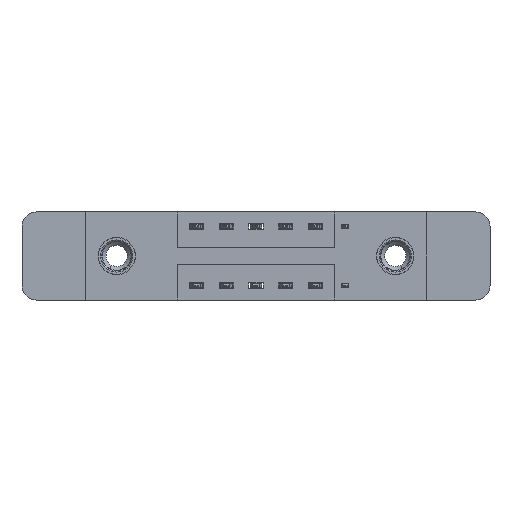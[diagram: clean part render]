
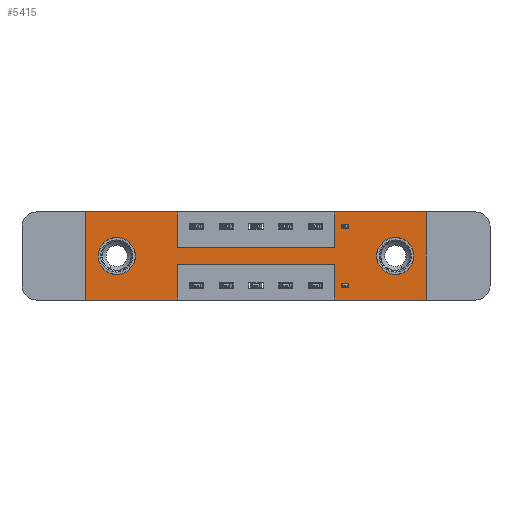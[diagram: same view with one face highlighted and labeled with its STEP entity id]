
A CAD part, front view. The second image highlights one B-rep face of the part: STEP entity #5415.
In plain terms, the highlighted planar face has unit normal (0, -1, 0).
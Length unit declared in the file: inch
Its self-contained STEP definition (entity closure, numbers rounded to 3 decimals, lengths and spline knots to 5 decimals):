
#139 = LINE ( 'NONE', #3190, #13564 ) ;
#177 = CARTESIAN_POINT ( 'NONE',  ( 1.3025, 0., -0.107 ) ) ;
#240 = CARTESIAN_POINT ( 'NONE',  ( 0., 0., -0.37 ) ) ;
#278 = AXIS2_PLACEMENT_3D ( 'NONE', #502, #3787, #12575 ) ;
#338 = VECTOR ( 'NONE', #5071, 39.37008 ) ;
#409 = EDGE_CURVE ( 'NONE', #1438, #1711, #13217, .T. ) ;
#502 = CARTESIAN_POINT ( 'NONE',  ( 1.3025, 0., -0.185 ) ) ;
#896 = EDGE_CURVE ( 'NONE', #1711, #8041, #3485, .T. ) ;
#935 = EDGE_CURVE ( 'NONE', #6880, #13910, #6091, .T. ) ;
#1114 = DIRECTION ( 'NONE',  ( 0., 1., 0. ) ) ;
#1116 = LINE ( 'NONE', #10732, #1658 ) ;
#1154 = DIRECTION ( 'NONE',  ( 0., 0., -1. ) ) ;
#1238 = EDGE_CURVE ( 'NONE', #9080, #6046, #1116, .T. ) ;
#1250 = CARTESIAN_POINT ( 'NONE',  ( 0.3875, 0., -0.15 ) ) ;
#1273 = DIRECTION ( 'NONE',  ( 0., 0., -1. ) ) ;
#1438 = VERTEX_POINT ( 'NONE', #11184 ) ;
#1658 = VECTOR ( 'NONE', #5324, 39.37008 ) ;
#1711 = VERTEX_POINT ( 'NONE', #3855 ) ;
#1749 = VECTOR ( 'NONE', #9826, 39.37008 ) ;
#1819 = ORIENTED_EDGE ( 'NONE', *, *, #8376, .T. ) ;
#1899 = DIRECTION ( 'NONE',  ( 0., 1., 0. ) ) ;
#1933 = CARTESIAN_POINT ( 'NONE',  ( 0., 0., 0. ) ) ;
#2017 = EDGE_CURVE ( 'NONE', #7838, #10262, #11457, .T. ) ;
#2241 = CARTESIAN_POINT ( 'NONE',  ( 1.0475, 0., 0. ) ) ;
#2287 = CARTESIAN_POINT ( 'NONE',  ( 1.0475, 0., -0.15 ) ) ;
#2337 = ORIENTED_EDGE ( 'NONE', *, *, #7295, .T. ) ;
#2591 = DIRECTION ( 'NONE',  ( 1., 0., 0. ) ) ;
#2767 = CARTESIAN_POINT ( 'NONE',  ( 1.435, 0., -0.37 ) ) ;
#2773 = EDGE_CURVE ( 'NONE', #8041, #6880, #8768, .T. ) ;
#2799 = EDGE_CURVE ( 'NONE', #12626, #1438, #139, .T. ) ;
#2966 = CARTESIAN_POINT ( 'NONE',  ( 1.3025, 0., -0.263 ) ) ;
#3064 = VERTEX_POINT ( 'NONE', #177 ) ;
#3154 = CARTESIAN_POINT ( 'NONE',  ( 0., 0., -0.37 ) ) ;
#3190 = CARTESIAN_POINT ( 'NONE',  ( 1.0475, 0., -0.37 ) ) ;
#3387 = LINE ( 'NONE', #240, #10781 ) ;
#3448 = VECTOR ( 'NONE', #5158, 39.37008 ) ;
#3485 = LINE ( 'NONE', #5408, #6715 ) ;
#3629 = DIRECTION ( 'NONE',  ( 0., 0., -1. ) ) ;
#3664 = VECTOR ( 'NONE', #6370, 39.37008 ) ;
#3766 = VERTEX_POINT ( 'NONE', #12826 ) ;
#3787 = DIRECTION ( 'NONE',  ( 0., 1., 0. ) ) ;
#3855 = CARTESIAN_POINT ( 'NONE',  ( 0.3875, 0., -0.22 ) ) ;
#3874 = CARTESIAN_POINT ( 'NONE',  ( 1.0475, 0., -0.37 ) ) ;
#3991 = VECTOR ( 'NONE', #11404, 39.37008 ) ;
#3993 = EDGE_CURVE ( 'NONE', #3766, #13874, #11278, .T. ) ;
#4260 = CARTESIAN_POINT ( 'NONE',  ( 0.1325, 0., -0.263 ) ) ;
#4363 = AXIS2_PLACEMENT_3D ( 'NONE', #8697, #1899, #12703 ) ;
#4497 = ORIENTED_EDGE ( 'NONE', *, *, #3993, .F. ) ;
#4551 = CARTESIAN_POINT ( 'NONE',  ( 1.3025, 0., -0.185 ) ) ;
#5003 = VECTOR ( 'NONE', #2591, 39.37008 ) ;
#5026 = AXIS2_PLACEMENT_3D ( 'NONE', #3154, #7511, #1154 ) ;
#5071 = DIRECTION ( 'NONE',  ( -1., 0., 0. ) ) ;
#5142 = EDGE_LOOP ( 'NONE', ( #1819, #2337 ) ) ;
#5158 = DIRECTION ( 'NONE',  ( 0., 0., -1. ) ) ;
#5266 = CIRCLE ( 'NONE', #4363, 0.078 ) ;
#5279 = FACE_BOUND ( 'NONE', #5142, .T. ) ;
#5324 = DIRECTION ( 'NONE',  ( 1., 0., 0. ) ) ;
#5398 = DIRECTION ( 'NONE',  ( 0., 0., 1. ) ) ;
#5408 = CARTESIAN_POINT ( 'NONE',  ( 0.3875, 0., -0.37 ) ) ;
#5415 = ADVANCED_FACE ( 'NONE', ( #5279, #11534, #9643 ), #12884, .T. ) ;
#5534 = ORIENTED_EDGE ( 'NONE', *, *, #2017, .T. ) ;
#5658 = CARTESIAN_POINT ( 'NONE',  ( 0.1325, 0., -0.107 ) ) ;
#6001 = VERTEX_POINT ( 'NONE', #2767 ) ;
#6046 = VERTEX_POINT ( 'NONE', #11636 ) ;
#6091 = LINE ( 'NONE', #6300, #8064 ) ;
#6149 = LINE ( 'NONE', #11495, #3448 ) ;
#6277 = DIRECTION ( 'NONE',  ( 1., 0., 0. ) ) ;
#6282 = CARTESIAN_POINT ( 'NONE',  ( 0.3875, 0., -0.22 ) ) ;
#6300 = CARTESIAN_POINT ( 'NONE',  ( 0., 0., 0. ) ) ;
#6370 = DIRECTION ( 'NONE',  ( 0., 0., 1. ) ) ;
#6399 = CIRCLE ( 'NONE', #278, 0.078 ) ;
#6680 = DIRECTION ( 'NONE',  ( 0., 0., 1. ) ) ;
#6715 = VECTOR ( 'NONE', #1273, 39.37008 ) ;
#6880 = VERTEX_POINT ( 'NONE', #13185 ) ;
#7243 = DIRECTION ( 'NONE',  ( 0., 0., 1. ) ) ;
#7295 = EDGE_CURVE ( 'NONE', #11156, #3064, #9133, .T. ) ;
#7344 = ORIENTED_EDGE ( 'NONE', *, *, #8258, .F. ) ;
#7386 = AXIS2_PLACEMENT_3D ( 'NONE', #9753, #1114, #6680 ) ;
#7466 = EDGE_CURVE ( 'NONE', #11814, #9080, #11769, .T. ) ;
#7511 = DIRECTION ( 'NONE',  ( 0., -1., 0. ) ) ;
#7545 = AXIS2_PLACEMENT_3D ( 'NONE', #4551, #12349, #3629 ) ;
#7838 = VERTEX_POINT ( 'NONE', #5658 ) ;
#8041 = VERTEX_POINT ( 'NONE', #8097 ) ;
#8064 = VECTOR ( 'NONE', #7243, 39.37008 ) ;
#8097 = CARTESIAN_POINT ( 'NONE',  ( 0.3875, 0., -0.37 ) ) ;
#8100 = LINE ( 'NONE', #1250, #5003 ) ;
#8208 = ORIENTED_EDGE ( 'NONE', *, *, #409, .F. ) ;
#8258 = EDGE_CURVE ( 'NONE', #13910, #3766, #9640, .T. ) ;
#8376 = EDGE_CURVE ( 'NONE', #3064, #11156, #6399, .T. ) ;
#8697 = CARTESIAN_POINT ( 'NONE',  ( 0.1325, 0., -0.185 ) ) ;
#8768 = LINE ( 'NONE', #12122, #1749 ) ;
#8789 = ORIENTED_EDGE ( 'NONE', *, *, #896, .F. ) ;
#8815 = ORIENTED_EDGE ( 'NONE', *, *, #2799, .F. ) ;
#8833 = EDGE_CURVE ( 'NONE', #6046, #6001, #6149, .T. ) ;
#9024 = CARTESIAN_POINT ( 'NONE',  ( 0.3875, 0., 0. ) ) ;
#9080 = VERTEX_POINT ( 'NONE', #11894 ) ;
#9133 = CIRCLE ( 'NONE', #7545, 0.078 ) ;
#9161 = ORIENTED_EDGE ( 'NONE', *, *, #2773, .F. ) ;
#9181 = EDGE_CURVE ( 'NONE', #13874, #11814, #8100, .T. ) ;
#9329 = ORIENTED_EDGE ( 'NONE', *, *, #10178, .T. ) ;
#9640 = LINE ( 'NONE', #1933, #12511 ) ;
#9643 = FACE_OUTER_BOUND ( 'NONE', #11078, .T. ) ;
#9753 = CARTESIAN_POINT ( 'NONE',  ( 0.1325, 0., -0.185 ) ) ;
#9826 = DIRECTION ( 'NONE',  ( -1., 0., 0. ) ) ;
#9962 = ORIENTED_EDGE ( 'NONE', *, *, #935, .F. ) ;
#10178 = EDGE_CURVE ( 'NONE', #10262, #7838, #5266, .T. ) ;
#10262 = VERTEX_POINT ( 'NONE', #4260 ) ;
#10732 = CARTESIAN_POINT ( 'NONE',  ( 0., 0., 0. ) ) ;
#10781 = VECTOR ( 'NONE', #13240, 39.37008 ) ;
#11078 = EDGE_LOOP ( 'NONE', ( #8789, #8208, #8815, #13078, #13149, #12289, #12920, #11941, #4497, #7344, #9962, #9161 ) ) ;
#11156 = VERTEX_POINT ( 'NONE', #2966 ) ;
#11184 = CARTESIAN_POINT ( 'NONE',  ( 1.0475, 0., -0.22 ) ) ;
#11278 = LINE ( 'NONE', #9024, #3991 ) ;
#11404 = DIRECTION ( 'NONE',  ( 0., 0., -1. ) ) ;
#11457 = CIRCLE ( 'NONE', #7386, 0.078 ) ;
#11495 = CARTESIAN_POINT ( 'NONE',  ( 1.435, 0., 0. ) ) ;
#11534 = FACE_BOUND ( 'NONE', #13447, .T. ) ;
#11636 = CARTESIAN_POINT ( 'NONE',  ( 1.435, 0., 0. ) ) ;
#11769 = LINE ( 'NONE', #2241, #3664 ) ;
#11814 = VERTEX_POINT ( 'NONE', #2287 ) ;
#11894 = CARTESIAN_POINT ( 'NONE',  ( 1.0475, 0., 0. ) ) ;
#11941 = ORIENTED_EDGE ( 'NONE', *, *, #9181, .F. ) ;
#12024 = CARTESIAN_POINT ( 'NONE',  ( 0., 0., 0. ) ) ;
#12122 = CARTESIAN_POINT ( 'NONE',  ( 0., 0., -0.37 ) ) ;
#12289 = ORIENTED_EDGE ( 'NONE', *, *, #1238, .F. ) ;
#12349 = DIRECTION ( 'NONE',  ( 0., 1., 0. ) ) ;
#12511 = VECTOR ( 'NONE', #6277, 39.37008 ) ;
#12575 = DIRECTION ( 'NONE',  ( 0., 0., -1. ) ) ;
#12626 = VERTEX_POINT ( 'NONE', #3874 ) ;
#12703 = DIRECTION ( 'NONE',  ( 0., 0., 1. ) ) ;
#12826 = CARTESIAN_POINT ( 'NONE',  ( 0.3875, 0., 0. ) ) ;
#12884 = PLANE ( 'NONE',  #5026 ) ;
#12901 = EDGE_CURVE ( 'NONE', #6001, #12626, #3387, .T. ) ;
#12920 = ORIENTED_EDGE ( 'NONE', *, *, #7466, .F. ) ;
#13078 = ORIENTED_EDGE ( 'NONE', *, *, #12901, .F. ) ;
#13149 = ORIENTED_EDGE ( 'NONE', *, *, #8833, .F. ) ;
#13185 = CARTESIAN_POINT ( 'NONE',  ( 0., 0., -0.37 ) ) ;
#13217 = LINE ( 'NONE', #6282, #338 ) ;
#13240 = DIRECTION ( 'NONE',  ( -1., 0., 0. ) ) ;
#13447 = EDGE_LOOP ( 'NONE', ( #5534, #9329 ) ) ;
#13564 = VECTOR ( 'NONE', #5398, 39.37008 ) ;
#13874 = VERTEX_POINT ( 'NONE', #14039 ) ;
#13910 = VERTEX_POINT ( 'NONE', #12024 ) ;
#14039 = CARTESIAN_POINT ( 'NONE',  ( 0.3875, 0., -0.15 ) ) ;
